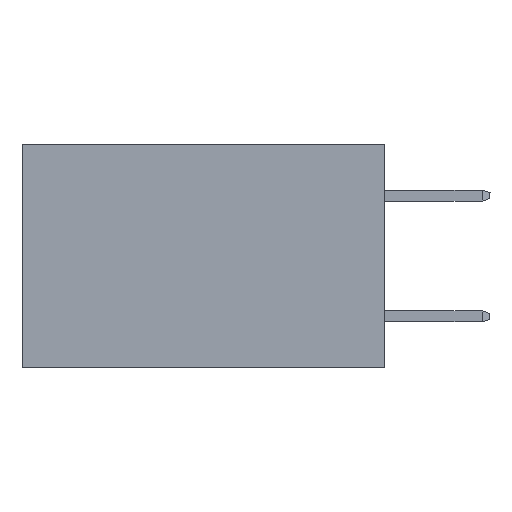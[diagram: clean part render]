
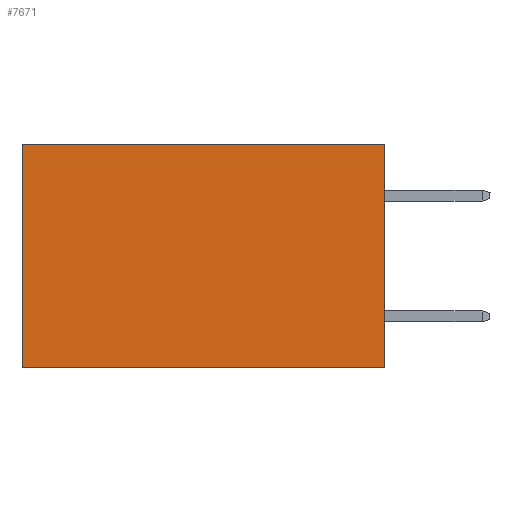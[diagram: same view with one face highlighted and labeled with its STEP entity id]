
A CAD part, left-side view. The second image highlights one B-rep face of the part: STEP entity #7671.
In plain terms, the highlighted planar face has unit normal (-1, 0, 0).
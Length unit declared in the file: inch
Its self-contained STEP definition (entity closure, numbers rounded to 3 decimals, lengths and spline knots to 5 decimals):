
#1231 = CARTESIAN_POINT ( 'NONE',  ( 0.298, 0.6, 0. ) ) ;
#1512 = ORIENTED_EDGE ( 'NONE', *, *, #6446, .F. ) ;
#1808 = CARTESIAN_POINT ( 'NONE',  ( 0.298, 0., -0.37 ) ) ;
#1861 = FACE_OUTER_BOUND ( 'NONE', #5193, .T. ) ;
#1918 = LINE ( 'NONE', #1231, #19004 ) ;
#2843 = DIRECTION ( 'NONE',  ( 0., 0., -1. ) ) ;
#3348 = VERTEX_POINT ( 'NONE', #9715 ) ;
#3444 = VECTOR ( 'NONE', #17277, 39.37008 ) ;
#4787 = VERTEX_POINT ( 'NONE', #18228 ) ;
#5193 = EDGE_LOOP ( 'NONE', ( #20082, #21391, #1512, #12902 ) ) ;
#6296 = LINE ( 'NONE', #15608, #3444 ) ;
#6446 = EDGE_CURVE ( 'NONE', #14521, #3348, #19251, .T. ) ;
#6987 = DIRECTION ( 'NONE',  ( 1., 0., 0. ) ) ;
#7671 = ADVANCED_FACE ( 'NONE', ( #1861 ), #10500, .F. ) ;
#7842 = CARTESIAN_POINT ( 'NONE',  ( 0.298, 0., 0. ) ) ;
#9715 = CARTESIAN_POINT ( 'NONE',  ( 0.298, 0., -0.37 ) ) ;
#10500 = PLANE ( 'NONE',  #13953 ) ;
#10618 = VERTEX_POINT ( 'NONE', #20515 ) ;
#12571 = LINE ( 'NONE', #1808, #13842 ) ;
#12681 = DIRECTION ( 'NONE',  ( 0., 0., -1. ) ) ;
#12902 = ORIENTED_EDGE ( 'NONE', *, *, #20413, .T. ) ;
#13386 = DIRECTION ( 'NONE',  ( 0., 1., 0. ) ) ;
#13842 = VECTOR ( 'NONE', #13386, 39.37008 ) ;
#13953 = AXIS2_PLACEMENT_3D ( 'NONE', #20805, #6987, #15313 ) ;
#14521 = VERTEX_POINT ( 'NONE', #7842 ) ;
#15313 = DIRECTION ( 'NONE',  ( 0., 0., -1. ) ) ;
#15608 = CARTESIAN_POINT ( 'NONE',  ( 0.298, 0., 0. ) ) ;
#17277 = DIRECTION ( 'NONE',  ( 0., 1., 0. ) ) ;
#17709 = VECTOR ( 'NONE', #2843, 39.37008 ) ;
#18228 = CARTESIAN_POINT ( 'NONE',  ( 0.298, 0.6, -0.37 ) ) ;
#19004 = VECTOR ( 'NONE', #12681, 39.37008 ) ;
#19119 = EDGE_CURVE ( 'NONE', #3348, #4787, #12571, .T. ) ;
#19251 = LINE ( 'NONE', #21008, #17709 ) ;
#20082 = ORIENTED_EDGE ( 'NONE', *, *, #20126, .T. ) ;
#20126 = EDGE_CURVE ( 'NONE', #10618, #4787, #1918, .T. ) ;
#20413 = EDGE_CURVE ( 'NONE', #14521, #10618, #6296, .T. ) ;
#20515 = CARTESIAN_POINT ( 'NONE',  ( 0.298, 0.6, 0. ) ) ;
#20805 = CARTESIAN_POINT ( 'NONE',  ( 0.298, 0., 0. ) ) ;
#21008 = CARTESIAN_POINT ( 'NONE',  ( 0.298, 0., 0. ) ) ;
#21391 = ORIENTED_EDGE ( 'NONE', *, *, #19119, .F. ) ;
